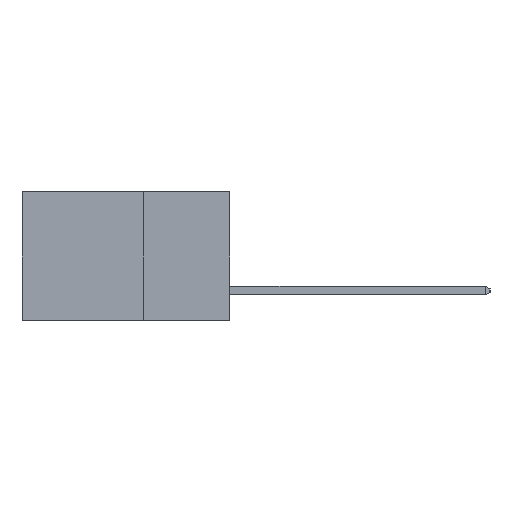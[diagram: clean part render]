
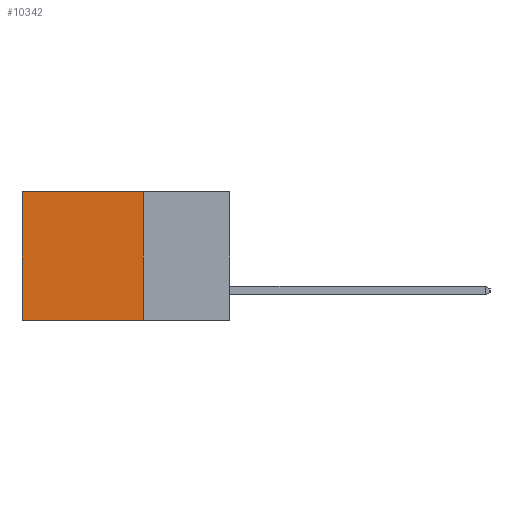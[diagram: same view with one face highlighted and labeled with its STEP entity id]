
A CAD part, left-side view. The second image highlights one B-rep face of the part: STEP entity #10342.
In plain terms, the highlighted planar face has unit normal (-1, 0, 0).
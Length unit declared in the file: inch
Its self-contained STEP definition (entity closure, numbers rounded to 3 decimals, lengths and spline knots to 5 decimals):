
#145 = VECTOR ( 'NONE', #2360, 39.37008 ) ;
#205 = ORIENTED_EDGE ( 'NONE', *, *, #8618, .T. ) ;
#209 = ORIENTED_EDGE ( 'NONE', *, *, #1467, .F. ) ;
#268 = ORIENTED_EDGE ( 'NONE', *, *, #9381, .F. ) ;
#328 = ORIENTED_EDGE ( 'NONE', *, *, #5917, .T. ) ;
#814 = EDGE_LOOP ( 'NONE', ( #205, #209, #268, #328 ) ) ;
#1114 = VERTEX_POINT ( 'NONE', #8717 ) ;
#1349 = CARTESIAN_POINT ( 'NONE',  ( 0.2615, 0.25, -0.37 ) ) ;
#1467 = EDGE_CURVE ( 'NONE', #2798, #1114, #3240, .T. ) ;
#1740 = DIRECTION ( 'NONE',  ( 1., 0., 0. ) ) ;
#2360 = DIRECTION ( 'NONE',  ( 0., 0., -1. ) ) ;
#2496 = DIRECTION ( 'NONE',  ( 0., 1., 0. ) ) ;
#2620 = CARTESIAN_POINT ( 'NONE',  ( 0.2615, 0.6, 0. ) ) ;
#2798 = VERTEX_POINT ( 'NONE', #5239 ) ;
#3159 = DIRECTION ( 'NONE',  ( 0., 1., 0. ) ) ;
#3240 = LINE ( 'NONE', #10819, #4858 ) ;
#4245 = VERTEX_POINT ( 'NONE', #2620 ) ;
#4858 = VECTOR ( 'NONE', #2496, 39.37008 ) ;
#5239 = CARTESIAN_POINT ( 'NONE',  ( 0.2615, 0.25, -0.37 ) ) ;
#5917 = EDGE_CURVE ( 'NONE', #8151, #4245, #10901, .T. ) ;
#6881 = VECTOR ( 'NONE', #3159, 39.37008 ) ;
#7250 = CARTESIAN_POINT ( 'NONE',  ( 0.2615, 0.25, 0. ) ) ;
#7334 = CARTESIAN_POINT ( 'NONE',  ( 0.2615, 0.25, -0.37 ) ) ;
#7713 = LINE ( 'NONE', #1349, #145 ) ;
#8150 = DIRECTION ( 'NONE',  ( 0., 0., -1. ) ) ;
#8151 = VERTEX_POINT ( 'NONE', #7250 ) ;
#8586 = CARTESIAN_POINT ( 'NONE',  ( 0.2615, 0.6, -0.37 ) ) ;
#8618 = EDGE_CURVE ( 'NONE', #4245, #1114, #11445, .T. ) ;
#8717 = CARTESIAN_POINT ( 'NONE',  ( 0.2615, 0.6, -0.37 ) ) ;
#9013 = AXIS2_PLACEMENT_3D ( 'NONE', #7334, #1740, #8150 ) ;
#9065 = FACE_OUTER_BOUND ( 'NONE', #814, .T. ) ;
#9311 = VECTOR ( 'NONE', #11036, 39.37008 ) ;
#9381 = EDGE_CURVE ( 'NONE', #8151, #2798, #7713, .T. ) ;
#10073 = CARTESIAN_POINT ( 'NONE',  ( 0.2615, 0.25, 0. ) ) ;
#10342 = ADVANCED_FACE ( 'NONE', ( #9065 ), #10503, .F. ) ;
#10503 = PLANE ( 'NONE',  #9013 ) ;
#10819 = CARTESIAN_POINT ( 'NONE',  ( 0.2615, 0.25, -0.37 ) ) ;
#10901 = LINE ( 'NONE', #10073, #6881 ) ;
#11036 = DIRECTION ( 'NONE',  ( 0., 0., -1. ) ) ;
#11445 = LINE ( 'NONE', #8586, #9311 ) ;
